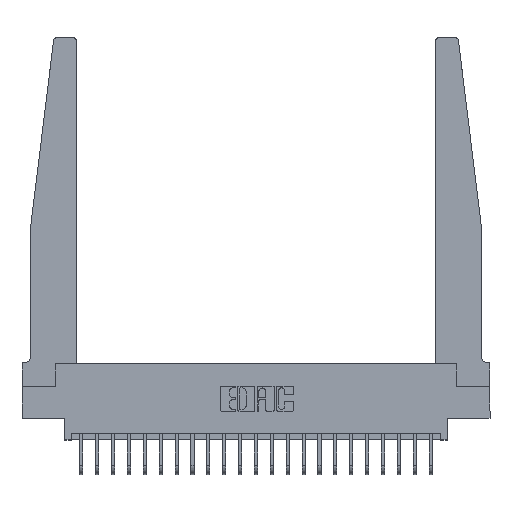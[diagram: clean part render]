
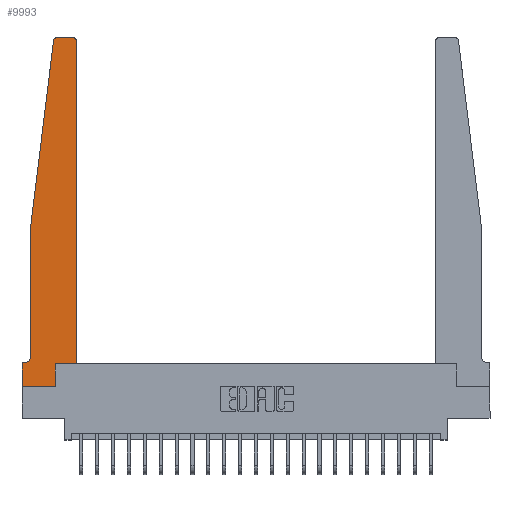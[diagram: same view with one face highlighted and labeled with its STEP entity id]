
A CAD part, top view. The second image highlights one B-rep face of the part: STEP entity #9993.
In plain terms, the highlighted planar face has unit normal (0, 0, 1).
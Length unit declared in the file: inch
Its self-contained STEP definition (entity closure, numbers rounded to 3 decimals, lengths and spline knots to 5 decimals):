
#213 = AXIS2_PLACEMENT_3D ( 'NONE', #16857, #1238, #8905 ) ;
#244 = CARTESIAN_POINT ( 'NONE',  ( 0.425, 0.18, 0.37 ) ) ;
#1238 = DIRECTION ( 'NONE',  ( 0., 0., 1. ) ) ;
#1425 = CIRCLE ( 'NONE', #7056, 0.05 ) ;
#1500 = VECTOR ( 'NONE', #12347, 39.37008 ) ;
#1636 = VECTOR ( 'NONE', #7942, 39.37008 ) ;
#1772 = EDGE_CURVE ( 'NONE', #23787, #11770, #14221, .T. ) ;
#1792 = VERTEX_POINT ( 'NONE', #10004 ) ;
#1877 = EDGE_CURVE ( 'NONE', #10758, #3121, #12970, .T. ) ;
#1908 = VECTOR ( 'NONE', #23961, 39.37008 ) ;
#1948 = ORIENTED_EDGE ( 'NONE', *, *, #3053, .T. ) ;
#2229 = CARTESIAN_POINT ( 'NONE',  ( 0.2605, 0.18, 0.37 ) ) ;
#2345 = DIRECTION ( 'NONE',  ( -0.122, -0.992, 0. ) ) ;
#2551 = CIRCLE ( 'NONE', #8579, 0.03 ) ;
#2699 = EDGE_CURVE ( 'NONE', #1792, #6391, #7432, .T. ) ;
#2851 = VERTEX_POINT ( 'NONE', #2229 ) ;
#3053 = EDGE_CURVE ( 'NONE', #6391, #10758, #19849, .T. ) ;
#3121 = VERTEX_POINT ( 'NONE', #14107 ) ;
#3222 = ORIENTED_EDGE ( 'NONE', *, *, #1772, .T. ) ;
#3295 = PLANE ( 'NONE',  #21800 ) ;
#3828 = ORIENTED_EDGE ( 'NONE', *, *, #11761, .T. ) ;
#4150 = DIRECTION ( 'NONE',  ( 0., 0., -1. ) ) ;
#4208 = VERTEX_POINT ( 'NONE', #8337 ) ;
#4794 = LINE ( 'NONE', #23759, #14067 ) ;
#4935 = ORIENTED_EDGE ( 'NONE', *, *, #21368, .T. ) ;
#5035 = LINE ( 'NONE', #12378, #12074 ) ;
#5564 = CARTESIAN_POINT ( 'NONE',  ( 0., 0.1875, 0.37 ) ) ;
#5694 = LINE ( 'NONE', #20782, #7867 ) ;
#6391 = VERTEX_POINT ( 'NONE', #18476 ) ;
#6628 = ORIENTED_EDGE ( 'NONE', *, *, #11799, .T. ) ;
#7056 = AXIS2_PLACEMENT_3D ( 'NONE', #15505, #4150, #9897 ) ;
#7311 = DIRECTION ( 'NONE',  ( 0., 1., 0. ) ) ;
#7432 = CIRCLE ( 'NONE', #213, 0.03 ) ;
#7458 = EDGE_CURVE ( 'NONE', #11770, #21960, #2551, .T. ) ;
#7532 = VERTEX_POINT ( 'NONE', #10830 ) ;
#7867 = VECTOR ( 'NONE', #13290, 39.37008 ) ;
#7942 = DIRECTION ( 'NONE',  ( 0., -1., 0. ) ) ;
#8337 = CARTESIAN_POINT ( 'NONE',  ( 0., 0., 0.37 ) ) ;
#8460 = ORIENTED_EDGE ( 'NONE', *, *, #2699, .T. ) ;
#8579 = AXIS2_PLACEMENT_3D ( 'NONE', #20560, #18922, #16674 ) ;
#8690 = CARTESIAN_POINT ( 'NONE',  ( 0., 0.1875, 0.37 ) ) ;
#8905 = DIRECTION ( 'NONE',  ( 1., 0., 0. ) ) ;
#9300 = VERTEX_POINT ( 'NONE', #9397 ) ;
#9397 = CARTESIAN_POINT ( 'NONE',  ( 0.2605, 0., 0.37 ) ) ;
#9461 = VECTOR ( 'NONE', #9528, 39.37008 ) ;
#9528 = DIRECTION ( 'NONE',  ( 1., 0., 0. ) ) ;
#9809 = CARTESIAN_POINT ( 'NONE',  ( 0., 0., 0.37 ) ) ;
#9897 = DIRECTION ( 'NONE',  ( -1., 0., 0. ) ) ;
#9993 = ADVANCED_FACE ( 'NONE', ( #20411 ), #3295, .T. ) ;
#10004 = CARTESIAN_POINT ( 'NONE',  ( 0.27653, 2.75, 0.37 ) ) ;
#10017 = EDGE_CURVE ( 'NONE', #7532, #20863, #5694, .T. ) ;
#10139 = CARTESIAN_POINT ( 'NONE',  ( 0.065, 1.25, 0.37 ) ) ;
#10428 = ORIENTED_EDGE ( 'NONE', *, *, #10017, .T. ) ;
#10504 = ORIENTED_EDGE ( 'NONE', *, *, #19278, .T. ) ;
#10560 = ORIENTED_EDGE ( 'NONE', *, *, #1877, .T. ) ;
#10620 = CARTESIAN_POINT ( 'NONE',  ( 0.065, 1.25, 0.37 ) ) ;
#10758 = VERTEX_POINT ( 'NONE', #10139 ) ;
#10830 = CARTESIAN_POINT ( 'NONE',  ( 0.015, 0.1875, 0.37 ) ) ;
#11082 = EDGE_LOOP ( 'NONE', ( #10504, #8460, #1948, #10560, #3828, #10428, #22940, #4935, #23236, #6628, #3222, #13819 ) ) ;
#11761 = EDGE_CURVE ( 'NONE', #3121, #7532, #1425, .T. ) ;
#11770 = VERTEX_POINT ( 'NONE', #13757 ) ;
#11799 = EDGE_CURVE ( 'NONE', #2851, #23787, #15385, .T. ) ;
#12074 = VECTOR ( 'NONE', #19999, 39.37008 ) ;
#12347 = DIRECTION ( 'NONE',  ( 0., 1., 0. ) ) ;
#12378 = CARTESIAN_POINT ( 'NONE',  ( 0., 0., 0.37 ) ) ;
#12401 = DIRECTION ( 'NONE',  ( -1., 0., 0. ) ) ;
#12919 = DIRECTION ( 'NONE',  ( 1., 0., 0. ) ) ;
#12924 = LINE ( 'NONE', #9809, #1636 ) ;
#12970 = LINE ( 'NONE', #10620, #1908 ) ;
#13281 = LINE ( 'NONE', #22646, #18410 ) ;
#13290 = DIRECTION ( 'NONE',  ( -1., 0., 0. ) ) ;
#13757 = CARTESIAN_POINT ( 'NONE',  ( 0.425, 2.72, 0.37 ) ) ;
#13819 = ORIENTED_EDGE ( 'NONE', *, *, #7458, .T. ) ;
#14067 = VECTOR ( 'NONE', #12401, 39.37008 ) ;
#14107 = CARTESIAN_POINT ( 'NONE',  ( 0.065, 0.2375, 0.37 ) ) ;
#14221 = LINE ( 'NONE', #23454, #1500 ) ;
#15385 = LINE ( 'NONE', #244, #9461 ) ;
#15423 = VECTOR ( 'NONE', #2345, 39.37008 ) ;
#15505 = CARTESIAN_POINT ( 'NONE',  ( 0.015, 0.2375, 0.37 ) ) ;
#16674 = DIRECTION ( 'NONE',  ( 1., 0., 0. ) ) ;
#16857 = CARTESIAN_POINT ( 'NONE',  ( 0.27653, 2.72, 0.37 ) ) ;
#17020 = DIRECTION ( 'NONE',  ( 0., 0., 1. ) ) ;
#17811 = EDGE_CURVE ( 'NONE', #20863, #4208, #12924, .T. ) ;
#18410 = VECTOR ( 'NONE', #7311, 39.37008 ) ;
#18476 = CARTESIAN_POINT ( 'NONE',  ( 0.24675, 2.72367, 0.37 ) ) ;
#18922 = DIRECTION ( 'NONE',  ( 0., 0., 1. ) ) ;
#19278 = EDGE_CURVE ( 'NONE', #21960, #1792, #4794, .T. ) ;
#19479 = CARTESIAN_POINT ( 'NONE',  ( 0.065, 1.25, 0.37 ) ) ;
#19849 = LINE ( 'NONE', #19479, #15423 ) ;
#19999 = DIRECTION ( 'NONE',  ( 1., 0., 0. ) ) ;
#20411 = FACE_OUTER_BOUND ( 'NONE', #11082, .T. ) ;
#20560 = CARTESIAN_POINT ( 'NONE',  ( 0.395, 2.72, 0.37 ) ) ;
#20782 = CARTESIAN_POINT ( 'NONE',  ( 0.065, 0.1875, 0.37 ) ) ;
#20863 = VERTEX_POINT ( 'NONE', #8690 ) ;
#20996 = EDGE_CURVE ( 'NONE', #9300, #2851, #13281, .T. ) ;
#21054 = CARTESIAN_POINT ( 'NONE',  ( 0.425, 0.18, 0.37 ) ) ;
#21368 = EDGE_CURVE ( 'NONE', #4208, #9300, #5035, .T. ) ;
#21789 = CARTESIAN_POINT ( 'NONE',  ( 0.395, 2.75, 0.37 ) ) ;
#21800 = AXIS2_PLACEMENT_3D ( 'NONE', #5564, #17020, #12919 ) ;
#21960 = VERTEX_POINT ( 'NONE', #21789 ) ;
#22646 = CARTESIAN_POINT ( 'NONE',  ( 0.2605, 0.18, 0.37 ) ) ;
#22940 = ORIENTED_EDGE ( 'NONE', *, *, #17811, .T. ) ;
#23236 = ORIENTED_EDGE ( 'NONE', *, *, #20996, .T. ) ;
#23454 = CARTESIAN_POINT ( 'NONE',  ( 0.425, 0.18, 0.37 ) ) ;
#23759 = CARTESIAN_POINT ( 'NONE',  ( 0.25, 2.75, 0.37 ) ) ;
#23787 = VERTEX_POINT ( 'NONE', #21054 ) ;
#23961 = DIRECTION ( 'NONE',  ( 0., -1., 0. ) ) ;
